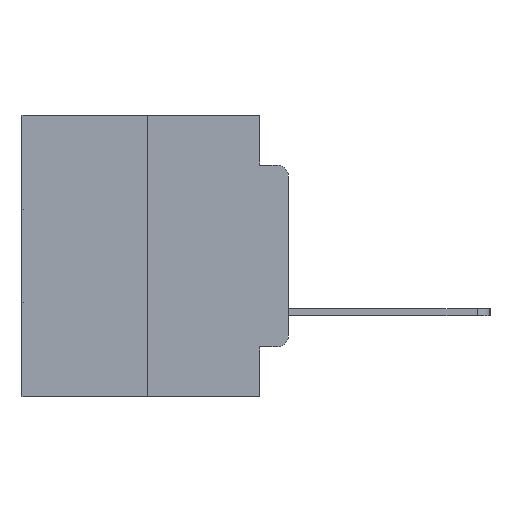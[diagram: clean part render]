
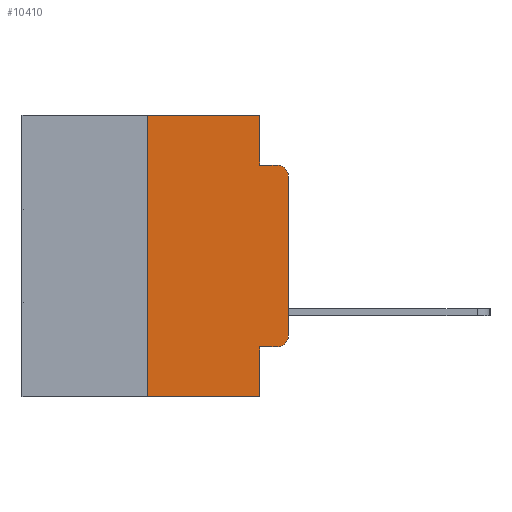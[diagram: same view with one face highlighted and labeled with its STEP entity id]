
A CAD part, left-side view. The second image highlights one B-rep face of the part: STEP entity #10410.
In plain terms, the highlighted planar face has unit normal (-1, 0, 0).
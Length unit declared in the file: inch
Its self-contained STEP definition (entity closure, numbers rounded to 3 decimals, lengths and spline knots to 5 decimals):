
#597 = LINE ( 'NONE', #15920, #22815 ) ;
#1614 = LINE ( 'NONE', #3444, #19483 ) ;
#1858 = EDGE_LOOP ( 'NONE', ( #3138, #9711, #16061, #5253, #5932, #18010, #13082, #2124, #19295, #14410 ) ) ;
#2124 = ORIENTED_EDGE ( 'NONE', *, *, #24182, .F. ) ;
#2373 = VECTOR ( 'NONE', #13262, 39.37008 ) ;
#3001 = CARTESIAN_POINT ( 'NONE',  ( 0., 0.051, -0.0885 ) ) ;
#3138 = ORIENTED_EDGE ( 'NONE', *, *, #17313, .T. ) ;
#3444 = CARTESIAN_POINT ( 'NONE',  ( 0., 0.473, -0.5 ) ) ;
#3650 = EDGE_CURVE ( 'NONE', #25303, #19813, #18419, .T. ) ;
#4228 = VERTEX_POINT ( 'NONE', #14512 ) ;
#4896 = EDGE_CURVE ( 'NONE', #18320, #10866, #25280, .T. ) ;
#5253 = ORIENTED_EDGE ( 'NONE', *, *, #12982, .F. ) ;
#5932 = ORIENTED_EDGE ( 'NONE', *, *, #4896, .F. ) ;
#6358 = DIRECTION ( 'NONE',  ( -1., 0., 0. ) ) ;
#6852 = VERTEX_POINT ( 'NONE', #22716 ) ;
#6937 = DIRECTION ( 'NONE',  ( 0., 0., -1. ) ) ;
#7132 = CARTESIAN_POINT ( 'NONE',  ( 0., 0.25, 0. ) ) ;
#7368 = LINE ( 'NONE', #19662, #12420 ) ;
#7774 = AXIS2_PLACEMENT_3D ( 'NONE', #19121, #6358, #21209 ) ;
#8414 = EDGE_CURVE ( 'NONE', #19813, #20977, #18600, .T. ) ;
#8967 = VERTEX_POINT ( 'NONE', #13393 ) ;
#9711 = ORIENTED_EDGE ( 'NONE', *, *, #14930, .T. ) ;
#10067 = AXIS2_PLACEMENT_3D ( 'NONE', #10203, #12362, #26939 ) ;
#10120 = CARTESIAN_POINT ( 'NONE',  ( 0., 0.473, 0. ) ) ;
#10203 = CARTESIAN_POINT ( 'NONE',  ( 0., 0.473, 0. ) ) ;
#10410 = ADVANCED_FACE ( 'NONE', ( #26928 ), #22832, .F. ) ;
#10866 = VERTEX_POINT ( 'NONE', #20040 ) ;
#11108 = CARTESIAN_POINT ( 'NONE',  ( 0., 0.051, 0. ) ) ;
#11135 = CARTESIAN_POINT ( 'NONE',  ( 0., 0., 0. ) ) ;
#12325 = VECTOR ( 'NONE', #23787, 39.37008 ) ;
#12362 = DIRECTION ( 'NONE',  ( 1., 0., 0. ) ) ;
#12420 = VECTOR ( 'NONE', #6937, 39.37008 ) ;
#12982 = EDGE_CURVE ( 'NONE', #10866, #20337, #7368, .T. ) ;
#13040 = CARTESIAN_POINT ( 'NONE',  ( 0., 0.25, 0. ) ) ;
#13082 = ORIENTED_EDGE ( 'NONE', *, *, #25084, .T. ) ;
#13262 = DIRECTION ( 'NONE',  ( 0., 0., -1. ) ) ;
#13393 = CARTESIAN_POINT ( 'NONE',  ( 0., 0.25, -0.5 ) ) ;
#13557 = LINE ( 'NONE', #7132, #24638 ) ;
#14368 = CARTESIAN_POINT ( 'NONE',  ( 0., 0.051, -0.5 ) ) ;
#14410 = ORIENTED_EDGE ( 'NONE', *, *, #8414, .T. ) ;
#14512 = CARTESIAN_POINT ( 'NONE',  ( 0., 0., -0.1085 ) ) ;
#14930 = EDGE_CURVE ( 'NONE', #4228, #6852, #18617, .T. ) ;
#15833 = EDGE_CURVE ( 'NONE', #20337, #6852, #597, .T. ) ;
#15920 = CARTESIAN_POINT ( 'NONE',  ( 0., 0.051, -0.0885 ) ) ;
#16061 = ORIENTED_EDGE ( 'NONE', *, *, #15833, .F. ) ;
#17123 = VECTOR ( 'NONE', #26856, 39.37008 ) ;
#17313 = EDGE_CURVE ( 'NONE', #20977, #4228, #23481, .T. ) ;
#18001 = DIRECTION ( 'NONE',  ( 0., -1., 0. ) ) ;
#18010 = ORIENTED_EDGE ( 'NONE', *, *, #26923, .F. ) ;
#18320 = VERTEX_POINT ( 'NONE', #13040 ) ;
#18419 = LINE ( 'NONE', #26940, #17123 ) ;
#18600 = CIRCLE ( 'NONE', #19401, 0.02 ) ;
#18617 = CIRCLE ( 'NONE', #7774, 0.02 ) ;
#19121 = CARTESIAN_POINT ( 'NONE',  ( 0., 0.02, -0.1085 ) ) ;
#19295 = ORIENTED_EDGE ( 'NONE', *, *, #3650, .T. ) ;
#19401 = AXIS2_PLACEMENT_3D ( 'NONE', #27452, #22953, #22741 ) ;
#19483 = VECTOR ( 'NONE', #26742, 39.37008 ) ;
#19662 = CARTESIAN_POINT ( 'NONE',  ( 0., 0.051, 0. ) ) ;
#19752 = VECTOR ( 'NONE', #22374, 39.37008 ) ;
#19813 = VERTEX_POINT ( 'NONE', #24574 ) ;
#20040 = CARTESIAN_POINT ( 'NONE',  ( 0., 0.051, 0. ) ) ;
#20337 = VERTEX_POINT ( 'NONE', #3001 ) ;
#20977 = VERTEX_POINT ( 'NONE', #22253 ) ;
#21209 = DIRECTION ( 'NONE',  ( 0., 0., -1. ) ) ;
#21945 = DIRECTION ( 'NONE',  ( 0., 0., 1. ) ) ;
#22253 = CARTESIAN_POINT ( 'NONE',  ( 0., 0., -0.3915 ) ) ;
#22374 = DIRECTION ( 'NONE',  ( 0., -1., 0. ) ) ;
#22716 = CARTESIAN_POINT ( 'NONE',  ( 0., 0.02, -0.0885 ) ) ;
#22741 = DIRECTION ( 'NONE',  ( 0., 0., -1. ) ) ;
#22815 = VECTOR ( 'NONE', #18001, 39.37008 ) ;
#22832 = PLANE ( 'NONE',  #10067 ) ;
#22953 = DIRECTION ( 'NONE',  ( -1., 0., 0. ) ) ;
#23342 = CARTESIAN_POINT ( 'NONE',  ( 0., 0.051, -0.4115 ) ) ;
#23481 = LINE ( 'NONE', #11135, #12325 ) ;
#23787 = DIRECTION ( 'NONE',  ( 0., 0., 1. ) ) ;
#24182 = EDGE_CURVE ( 'NONE', #25303, #26551, #25064, .T. ) ;
#24574 = CARTESIAN_POINT ( 'NONE',  ( 0., 0.02, -0.4115 ) ) ;
#24638 = VECTOR ( 'NONE', #21945, 39.37008 ) ;
#25064 = LINE ( 'NONE', #11108, #2373 ) ;
#25084 = EDGE_CURVE ( 'NONE', #8967, #26551, #1614, .T. ) ;
#25280 = LINE ( 'NONE', #10120, #19752 ) ;
#25303 = VERTEX_POINT ( 'NONE', #23342 ) ;
#26551 = VERTEX_POINT ( 'NONE', #14368 ) ;
#26742 = DIRECTION ( 'NONE',  ( 0., -1., 0. ) ) ;
#26856 = DIRECTION ( 'NONE',  ( 0., -1., 0. ) ) ;
#26923 = EDGE_CURVE ( 'NONE', #8967, #18320, #13557, .T. ) ;
#26928 = FACE_OUTER_BOUND ( 'NONE', #1858, .T. ) ;
#26939 = DIRECTION ( 'NONE',  ( 0., 0., -1. ) ) ;
#26940 = CARTESIAN_POINT ( 'NONE',  ( 0., 0.051, -0.4115 ) ) ;
#27452 = CARTESIAN_POINT ( 'NONE',  ( 0., 0.02, -0.3915 ) ) ;
